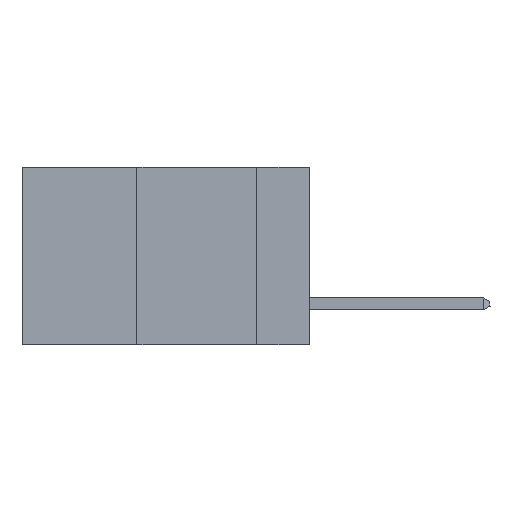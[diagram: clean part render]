
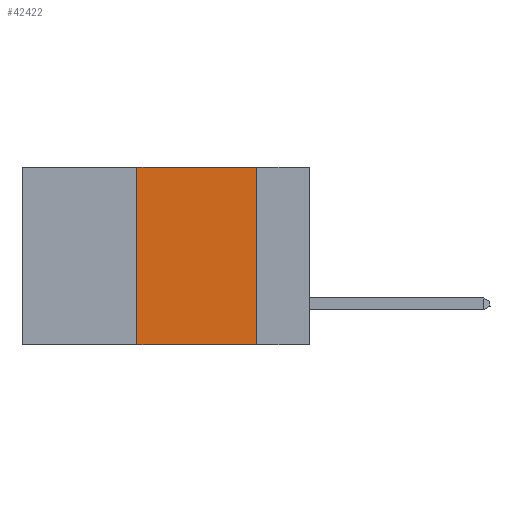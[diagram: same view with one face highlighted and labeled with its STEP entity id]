
A CAD part, left-side view. The second image highlights one B-rep face of the part: STEP entity #42422.
In plain terms, the highlighted planar face has unit normal (-1, 0, 0).
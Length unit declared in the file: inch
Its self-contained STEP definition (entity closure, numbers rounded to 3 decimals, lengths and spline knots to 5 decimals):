
#149 = EDGE_CURVE ( 'NONE', #41521, #48268, #15748, .T. ) ;
#3415 = LINE ( 'NONE', #17507, #14550 ) ;
#3576 = ORIENTED_EDGE ( 'NONE', *, *, #4943, .T. ) ;
#4842 = LINE ( 'NONE', #6498, #43532 ) ;
#4943 = EDGE_CURVE ( 'NONE', #41883, #16914, #4842, .T. ) ;
#5787 = VECTOR ( 'NONE', #25884, 39.37008 ) ;
#6498 = CARTESIAN_POINT ( 'NONE',  ( 0., 0.6, -0.37 ) ) ;
#9370 = ORIENTED_EDGE ( 'NONE', *, *, #13760, .F. ) ;
#9484 = EDGE_LOOP ( 'NONE', ( #19599, #12090, #9370, #3576 ) ) ;
#10603 = EDGE_CURVE ( 'NONE', #48268, #16914, #45243, .T. ) ;
#12090 = ORIENTED_EDGE ( 'NONE', *, *, #149, .F. ) ;
#13760 = EDGE_CURVE ( 'NONE', #41883, #41521, #3415, .T. ) ;
#14550 = VECTOR ( 'NONE', #29014, 39.37008 ) ;
#15181 = AXIS2_PLACEMENT_3D ( 'NONE', #40229, #44301, #48059 ) ;
#15748 = LINE ( 'NONE', #32940, #5787 ) ;
#16914 = VERTEX_POINT ( 'NONE', #40086 ) ;
#17507 = CARTESIAN_POINT ( 'NONE',  ( 0., 0.36, 0. ) ) ;
#19599 = ORIENTED_EDGE ( 'NONE', *, *, #10603, .F. ) ;
#25884 = DIRECTION ( 'NONE',  ( 0., -1., 0. ) ) ;
#26037 = CARTESIAN_POINT ( 'NONE',  ( 0., 0.11, 0. ) ) ;
#26556 = VECTOR ( 'NONE', #40273, 39.37008 ) ;
#29014 = DIRECTION ( 'NONE',  ( 0., 0., 1. ) ) ;
#32940 = CARTESIAN_POINT ( 'NONE',  ( 0., 0.6, 0. ) ) ;
#32944 = PLANE ( 'NONE',  #15181 ) ;
#35974 = FACE_OUTER_BOUND ( 'NONE', #9484, .T. ) ;
#36441 = CARTESIAN_POINT ( 'NONE',  ( 0., 0.36, 0. ) ) ;
#37017 = CARTESIAN_POINT ( 'NONE',  ( 0., 0.11, 0. ) ) ;
#40086 = CARTESIAN_POINT ( 'NONE',  ( 0., 0.11, -0.37 ) ) ;
#40229 = CARTESIAN_POINT ( 'NONE',  ( 0., 0.6, 0. ) ) ;
#40273 = DIRECTION ( 'NONE',  ( 0., 0., -1. ) ) ;
#41521 = VERTEX_POINT ( 'NONE', #36441 ) ;
#41883 = VERTEX_POINT ( 'NONE', #43910 ) ;
#42422 = ADVANCED_FACE ( 'NONE', ( #35974 ), #32944, .F. ) ;
#43532 = VECTOR ( 'NONE', #47731, 39.37008 ) ;
#43910 = CARTESIAN_POINT ( 'NONE',  ( 0., 0.36, -0.37 ) ) ;
#44301 = DIRECTION ( 'NONE',  ( 1., 0., 0. ) ) ;
#45243 = LINE ( 'NONE', #37017, #26556 ) ;
#47731 = DIRECTION ( 'NONE',  ( 0., -1., 0. ) ) ;
#48059 = DIRECTION ( 'NONE',  ( 0., 0., -1. ) ) ;
#48268 = VERTEX_POINT ( 'NONE', #26037 ) ;
